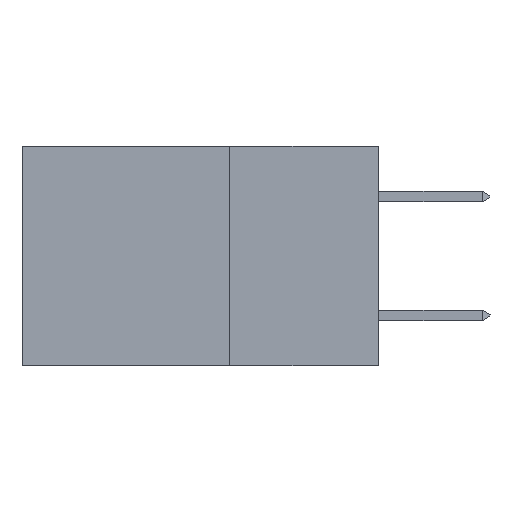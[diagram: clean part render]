
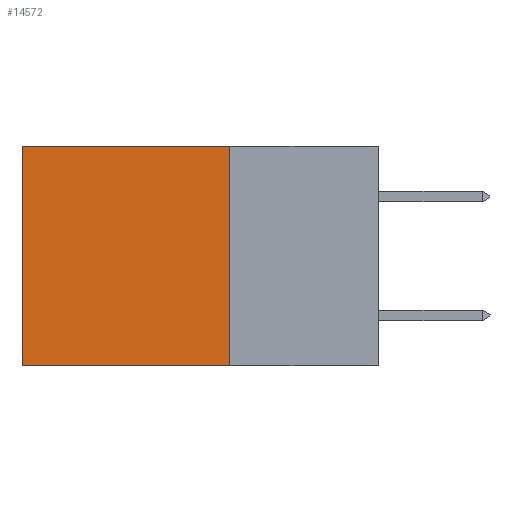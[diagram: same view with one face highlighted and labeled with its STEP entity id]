
A CAD part, left-side view. The second image highlights one B-rep face of the part: STEP entity #14572.
In plain terms, the highlighted planar face has unit normal (-1, 0, 0).
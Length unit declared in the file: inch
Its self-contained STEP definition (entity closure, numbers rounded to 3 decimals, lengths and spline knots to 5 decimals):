
#70 = DIRECTION ( 'NONE',  ( 0., 0., -1. ) ) ;
#605 = VERTEX_POINT ( 'NONE', #15025 ) ;
#2356 = VERTEX_POINT ( 'NONE', #20337 ) ;
#2444 = DIRECTION ( 'NONE',  ( 0., 0., -1. ) ) ;
#3284 = VECTOR ( 'NONE', #2444, 39.37008 ) ;
#3523 = CARTESIAN_POINT ( 'NONE',  ( 0.298, 0.25, 0. ) ) ;
#3529 = ORIENTED_EDGE ( 'NONE', *, *, #11504, .F. ) ;
#5706 = VECTOR ( 'NONE', #12753, 39.37008 ) ;
#5707 = VERTEX_POINT ( 'NONE', #9594 ) ;
#6665 = DIRECTION ( 'NONE',  ( 1., 0., 0. ) ) ;
#7823 = CARTESIAN_POINT ( 'NONE',  ( 0.298, 0.25, -0.37 ) ) ;
#8059 = EDGE_CURVE ( 'NONE', #5707, #2356, #8661, .T. ) ;
#8661 = LINE ( 'NONE', #16894, #12299 ) ;
#9295 = CARTESIAN_POINT ( 'NONE',  ( 0.298, 0.25, 0. ) ) ;
#9594 = CARTESIAN_POINT ( 'NONE',  ( 0.298, 0.6, 0. ) ) ;
#10114 = LINE ( 'NONE', #7823, #5706 ) ;
#10184 = EDGE_CURVE ( 'NONE', #17732, #2356, #10114, .T. ) ;
#10941 = EDGE_LOOP ( 'NONE', ( #17493, #20159, #3529, #17219 ) ) ;
#11504 = EDGE_CURVE ( 'NONE', #605, #17732, #12125, .T. ) ;
#12125 = LINE ( 'NONE', #9295, #3284 ) ;
#12299 = VECTOR ( 'NONE', #13487, 39.37008 ) ;
#12391 = AXIS2_PLACEMENT_3D ( 'NONE', #3523, #6665, #70 ) ;
#12692 = DIRECTION ( 'NONE',  ( 0., 1., 0. ) ) ;
#12753 = DIRECTION ( 'NONE',  ( 0., 1., 0. ) ) ;
#13268 = PLANE ( 'NONE',  #12391 ) ;
#13487 = DIRECTION ( 'NONE',  ( 0., 0., -1. ) ) ;
#14306 = CARTESIAN_POINT ( 'NONE',  ( 0.298, 0.25, 0. ) ) ;
#14572 = ADVANCED_FACE ( 'NONE', ( #15851 ), #13268, .F. ) ;
#15025 = CARTESIAN_POINT ( 'NONE',  ( 0.298, 0.25, 0. ) ) ;
#15851 = FACE_OUTER_BOUND ( 'NONE', #10941, .T. ) ;
#16894 = CARTESIAN_POINT ( 'NONE',  ( 0.298, 0.6, 0. ) ) ;
#17219 = ORIENTED_EDGE ( 'NONE', *, *, #19858, .T. ) ;
#17493 = ORIENTED_EDGE ( 'NONE', *, *, #8059, .T. ) ;
#17732 = VERTEX_POINT ( 'NONE', #21288 ) ;
#18592 = LINE ( 'NONE', #14306, #19093 ) ;
#19093 = VECTOR ( 'NONE', #12692, 39.37008 ) ;
#19858 = EDGE_CURVE ( 'NONE', #605, #5707, #18592, .T. ) ;
#20159 = ORIENTED_EDGE ( 'NONE', *, *, #10184, .F. ) ;
#20337 = CARTESIAN_POINT ( 'NONE',  ( 0.298, 0.6, -0.37 ) ) ;
#21288 = CARTESIAN_POINT ( 'NONE',  ( 0.298, 0.25, -0.37 ) ) ;
